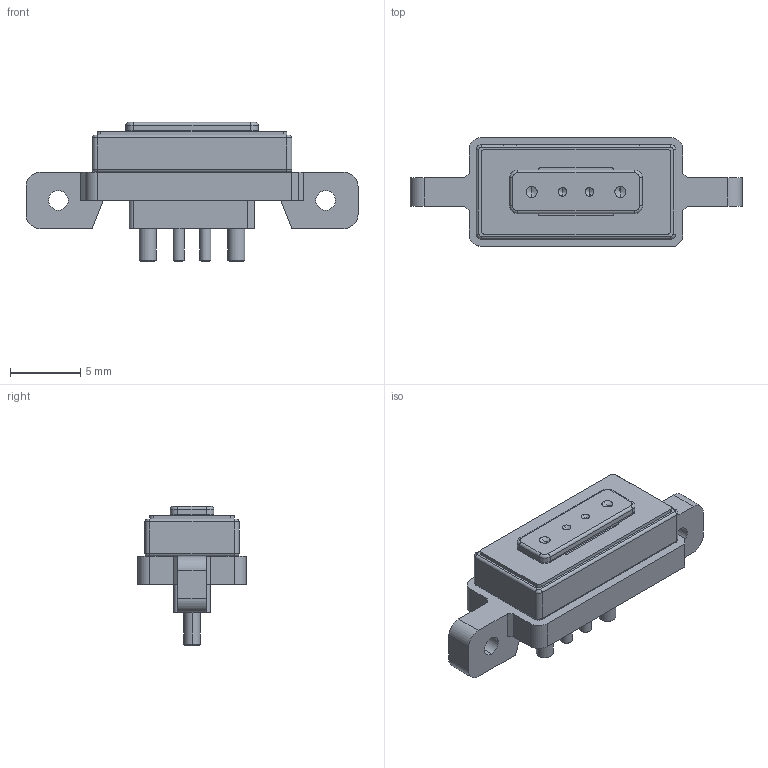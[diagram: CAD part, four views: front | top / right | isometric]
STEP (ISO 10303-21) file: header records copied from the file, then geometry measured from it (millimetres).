
FILE_DESCRIPTION (( 'STEP AP214' ), '1' );
FILE_NAME ('686D0432210123E.STEP', '2023-04-26T18:58:29', ( '' ), ( '' ), 'SwSTEP 2.0', 'SolidWorks 2020', '' );
FILE_SCHEMA (( 'AUTOMOTIVE_DESIGN' ));
Length unit declared in the file: millimetre
Products named in the file (1): 686D0432210123E
Bounding box: 23.6 x 7.7 x 9.9 mm (x, y, z)
Volume: 646.4 mm3; surface area: 974.4 mm2
Topology: 10 solids, 13 shells, 515 faces, 1406 edges, 904 vertices
Faces by surface type: plane 268, bspline 100, cylinder 99, cone 32, torus 16
Entity records: 21313 total; most frequent: CARTESIAN_POINT 8261, ORIENTED_EDGE 2780, DIRECTION 2251, EDGE_CURVE 1390, LINE 907, VECTOR 907, VERTEX_POINT 904, AXIS2_PLACEMENT_3D 672
